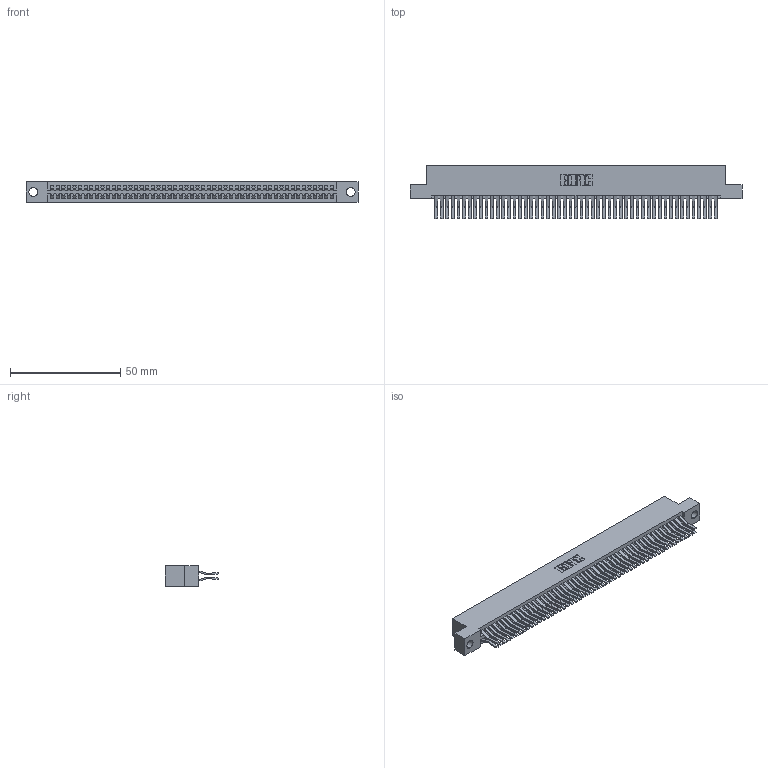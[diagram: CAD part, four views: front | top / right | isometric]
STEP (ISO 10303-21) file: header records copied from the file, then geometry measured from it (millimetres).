
FILE_DESCRIPTION (( 'STEP AP203' ), '1' );
FILE_NAME ('345-102-560-204.STEP', '2018-10-05T21:47:36', ( '' ), ( '' ), 'SwSTEP 2.0', 'SolidWorks 2016', '' );
FILE_SCHEMA (( 'CONFIG_CONTROL_DESIGN' ));
Length unit declared in the file: inch
Products named in the file (3): 345-102-560-204; 345-292-001_560 Tail; 345 Part_Flush Mounting Lugs - 0.156 Dia-TH
Assembly tree (103 placements, depth 2):
  345-102-560-204
    345 Part_Flush Mounting Lugs - 0.156 Dia-TH
    345-292-001_560 Tail  x102
Bounding box: 150.75 x 24.45 x 9.4 mm (x, y, z)
Volume: 15308.2 mm3; surface area: 24337 mm2
Topology: 103 solids, 103 shells, 5430 faces, 16151 edges, 10630 vertices
Faces by surface type: plane 3446, cylinder 1984
Entity records: 38895 total; most frequent: CARTESIAN_POINT 6512, ORIENTED_EDGE 6446, DIRECTION 5735, EDGE_CURVE 3223, VECTOR 2883, LINE 2883, VERTEX_POINT 2146, AXIS2_PLACEMENT_3D 1426
